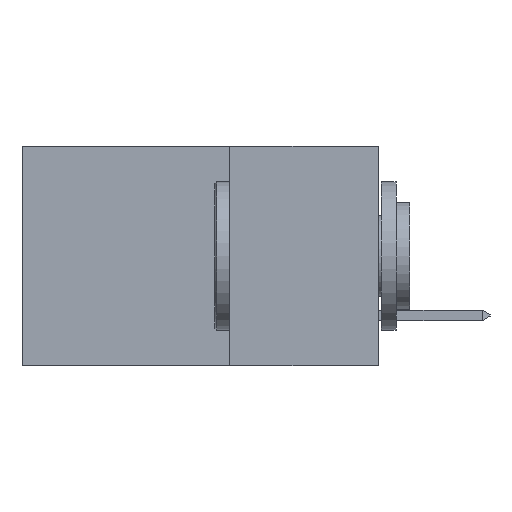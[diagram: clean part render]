
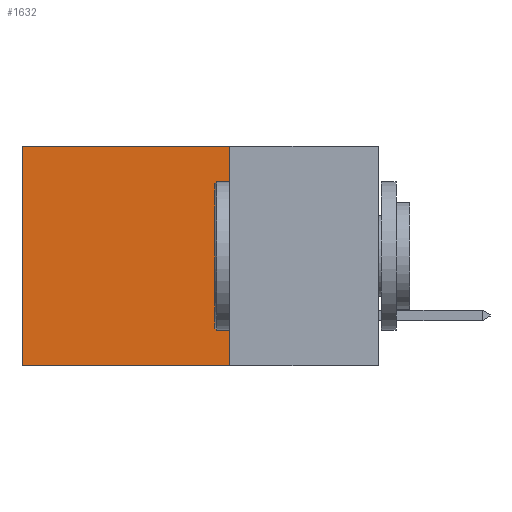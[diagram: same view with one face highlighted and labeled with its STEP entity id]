
A CAD part, left-side view. The second image highlights one B-rep face of the part: STEP entity #1632.
In plain terms, the highlighted planar face has unit normal (-1, 0, 0).
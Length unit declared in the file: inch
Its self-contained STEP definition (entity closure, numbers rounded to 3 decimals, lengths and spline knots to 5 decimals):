
#1252 = VECTOR ( 'NONE', #3615, 39.37008 ) ;
#1435 = AXIS2_PLACEMENT_3D ( 'NONE', #5603, #19141, #3717 ) ;
#1632 = ADVANCED_FACE ( 'NONE', ( #14856 ), #19080, .F. ) ;
#1974 = ORIENTED_EDGE ( 'NONE', *, *, #9228, .T. ) ;
#2946 = ORIENTED_EDGE ( 'NONE', *, *, #15845, .F. ) ;
#3464 = CARTESIAN_POINT ( 'NONE',  ( 0.2615, 0.25, -0.37 ) ) ;
#3511 = VERTEX_POINT ( 'NONE', #21320 ) ;
#3615 = DIRECTION ( 'NONE',  ( 0., 1., 0. ) ) ;
#3717 = DIRECTION ( 'NONE',  ( 0., 0., -1. ) ) ;
#4336 = VERTEX_POINT ( 'NONE', #19576 ) ;
#5603 = CARTESIAN_POINT ( 'NONE',  ( 0.2615, 0.25, -0.37 ) ) ;
#6138 = DIRECTION ( 'NONE',  ( 0., 0., -1. ) ) ;
#6203 = CARTESIAN_POINT ( 'NONE',  ( 0.2615, 0.25, -0.37 ) ) ;
#6262 = LINE ( 'NONE', #10507, #14979 ) ;
#6373 = LINE ( 'NONE', #3464, #1252 ) ;
#9228 = EDGE_CURVE ( 'NONE', #3511, #10487, #6262, .T. ) ;
#10172 = DIRECTION ( 'NONE',  ( 0., 0., -1. ) ) ;
#10487 = VERTEX_POINT ( 'NONE', #11299 ) ;
#10507 = CARTESIAN_POINT ( 'NONE',  ( 0.2615, 0.6, -0.37 ) ) ;
#10878 = EDGE_CURVE ( 'NONE', #13096, #4336, #15032, .T. ) ;
#11111 = DIRECTION ( 'NONE',  ( 0., 1., 0. ) ) ;
#11184 = CARTESIAN_POINT ( 'NONE',  ( 0.2615, 0.25, 0. ) ) ;
#11299 = CARTESIAN_POINT ( 'NONE',  ( 0.2615, 0.6, -0.37 ) ) ;
#11881 = CARTESIAN_POINT ( 'NONE',  ( 0.2615, 0.25, 0. ) ) ;
#11916 = ORIENTED_EDGE ( 'NONE', *, *, #13180, .T. ) ;
#12533 = EDGE_LOOP ( 'NONE', ( #1974, #2946, #15968, #11916 ) ) ;
#13096 = VERTEX_POINT ( 'NONE', #11881 ) ;
#13180 = EDGE_CURVE ( 'NONE', #13096, #3511, #21423, .T. ) ;
#13960 = VECTOR ( 'NONE', #6138, 39.37008 ) ;
#14856 = FACE_OUTER_BOUND ( 'NONE', #12533, .T. ) ;
#14979 = VECTOR ( 'NONE', #10172, 39.37008 ) ;
#15032 = LINE ( 'NONE', #6203, #13960 ) ;
#15845 = EDGE_CURVE ( 'NONE', #4336, #10487, #6373, .T. ) ;
#15968 = ORIENTED_EDGE ( 'NONE', *, *, #10878, .F. ) ;
#16477 = VECTOR ( 'NONE', #11111, 39.37008 ) ;
#19080 = PLANE ( 'NONE',  #1435 ) ;
#19141 = DIRECTION ( 'NONE',  ( 1., 0., 0. ) ) ;
#19576 = CARTESIAN_POINT ( 'NONE',  ( 0.2615, 0.25, -0.37 ) ) ;
#21320 = CARTESIAN_POINT ( 'NONE',  ( 0.2615, 0.6, 0. ) ) ;
#21423 = LINE ( 'NONE', #11184, #16477 ) ;
